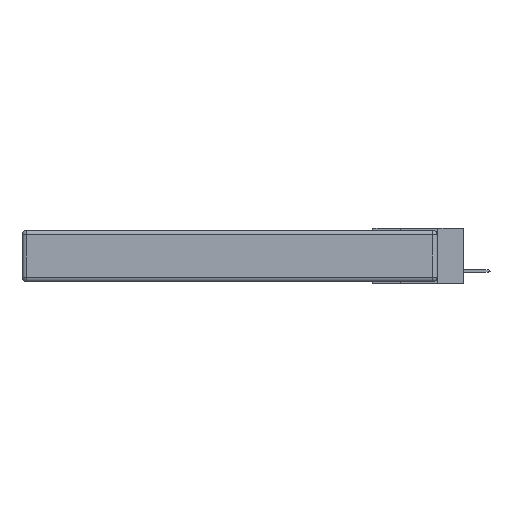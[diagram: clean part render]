
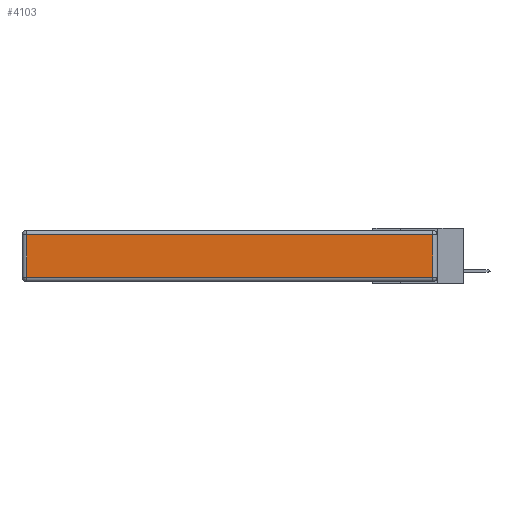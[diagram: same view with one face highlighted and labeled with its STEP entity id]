
A CAD part, left-side view. The second image highlights one B-rep face of the part: STEP entity #4103.
In plain terms, the highlighted planar face has unit normal (-1, 0, 0).
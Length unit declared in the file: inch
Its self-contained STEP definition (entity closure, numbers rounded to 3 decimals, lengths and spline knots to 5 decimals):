
#3174 = CARTESIAN_POINT ( 'NONE',  ( 0., 2.72, -0.313 ) ) ;
#3582 = CARTESIAN_POINT ( 'NONE',  ( 0., 2.72, -0.343 ) ) ;
#4103 = ADVANCED_FACE ( 'NONE', ( #14570 ), #6027, .T. ) ;
#4984 = AXIS2_PLACEMENT_3D ( 'NONE', #26709, #24113, #28762 ) ;
#5885 = CARTESIAN_POINT ( 'NONE',  ( 0., 2.72, -0.03 ) ) ;
#6027 = PLANE ( 'NONE',  #4984 ) ;
#7238 = VECTOR ( 'NONE', #9299, 39.37008 ) ;
#8089 = EDGE_LOOP ( 'NONE', ( #15038, #20670, #8126, #22207 ) ) ;
#8126 = ORIENTED_EDGE ( 'NONE', *, *, #9803, .T. ) ;
#8731 = VECTOR ( 'NONE', #16041, 39.37008 ) ;
#9299 = DIRECTION ( 'NONE',  ( 0., -1., 0. ) ) ;
#9417 = LINE ( 'NONE', #3582, #15083 ) ;
#9715 = DIRECTION ( 'NONE',  ( 0., 0., -1. ) ) ;
#9803 = EDGE_CURVE ( 'NONE', #16551, #16545, #14766, .T. ) ;
#9914 = CARTESIAN_POINT ( 'NONE',  ( 0., 0.03, -0.313 ) ) ;
#10535 = EDGE_CURVE ( 'NONE', #16545, #24799, #9417, .T. ) ;
#10999 = EDGE_CURVE ( 'NONE', #24807, #16551, #21448, .T. ) ;
#11669 = CARTESIAN_POINT ( 'NONE',  ( 0., 0., -0.313 ) ) ;
#14570 = FACE_OUTER_BOUND ( 'NONE', #8089, .T. ) ;
#14766 = LINE ( 'NONE', #17960, #17588 ) ;
#15038 = ORIENTED_EDGE ( 'NONE', *, *, #25142, .T. ) ;
#15083 = VECTOR ( 'NONE', #9715, 39.37008 ) ;
#16041 = DIRECTION ( 'NONE',  ( 0., 0., 1. ) ) ;
#16442 = LINE ( 'NONE', #11669, #7238 ) ;
#16545 = VERTEX_POINT ( 'NONE', #5885 ) ;
#16551 = VERTEX_POINT ( 'NONE', #23581 ) ;
#17588 = VECTOR ( 'NONE', #20253, 39.37008 ) ;
#17960 = CARTESIAN_POINT ( 'NONE',  ( 0., 2.75, -0.03 ) ) ;
#18675 = CARTESIAN_POINT ( 'NONE',  ( 0., 0.03, -0.343 ) ) ;
#20253 = DIRECTION ( 'NONE',  ( 0., 1., 0. ) ) ;
#20670 = ORIENTED_EDGE ( 'NONE', *, *, #10999, .T. ) ;
#21448 = LINE ( 'NONE', #18675, #8731 ) ;
#22207 = ORIENTED_EDGE ( 'NONE', *, *, #10535, .T. ) ;
#23581 = CARTESIAN_POINT ( 'NONE',  ( 0., 0.03, -0.03 ) ) ;
#24113 = DIRECTION ( 'NONE',  ( -1., 0., 0. ) ) ;
#24799 = VERTEX_POINT ( 'NONE', #3174 ) ;
#24807 = VERTEX_POINT ( 'NONE', #9914 ) ;
#25142 = EDGE_CURVE ( 'NONE', #24799, #24807, #16442, .T. ) ;
#26709 = CARTESIAN_POINT ( 'NONE',  ( 0., 0., -0.343 ) ) ;
#28762 = DIRECTION ( 'NONE',  ( 0., 0., 1. ) ) ;
